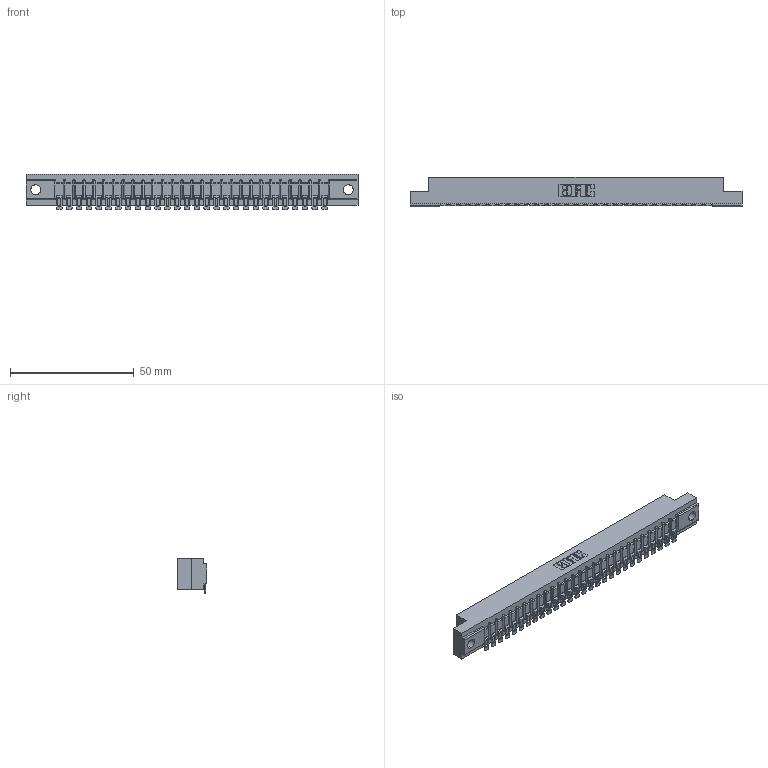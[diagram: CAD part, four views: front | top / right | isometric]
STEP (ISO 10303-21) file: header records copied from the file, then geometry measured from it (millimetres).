
FILE_DESCRIPTION (( 'STEP AP203' ), '1' );
FILE_NAME ('357-028-554-104.STEP', '2018-08-09T06:14:05', ( '' ), ( '' ), 'SwSTEP 2.0', 'SolidWorks 2016', '' );
FILE_SCHEMA (( 'CONFIG_CONTROL_DESIGN' ));
Length unit declared in the file: inch
Products named in the file (3): 307-290-002_554; 357-028-554-104; 307 Part_.156 Dia Mounting Holes
Assembly tree (29 placements, depth 2):
  357-028-554-104
    307 Part_.156 Dia Mounting Holes
    307-290-002_554  x28
Bounding box: 133.96 x 12.01 x 14.52 mm (x, y, z)
Volume: 14135.1 mm3; surface area: 17410.1 mm2
Topology: 29 solids, 29 shells, 2429 faces, 7443 edges, 4882 vertices
Faces by surface type: plane 1372, cylinder 999, sphere 58
Entity records: 27113 total; most frequent: CARTESIAN_POINT 4576, ORIENTED_EDGE 4564, DIRECTION 4450, EDGE_CURVE 2282, VECTOR 1742, LINE 1742, VERTEX_POINT 1480, AXIS2_PLACEMENT_3D 1354
